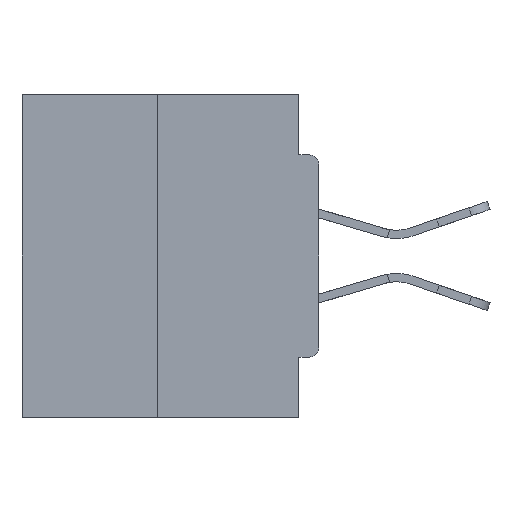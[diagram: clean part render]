
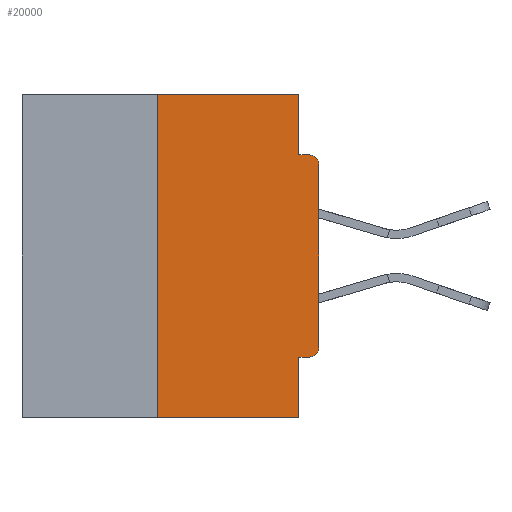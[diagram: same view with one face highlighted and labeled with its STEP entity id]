
A CAD part, left-side view. The second image highlights one B-rep face of the part: STEP entity #20000.
In plain terms, the highlighted planar face has unit normal (-1, 0, 0).
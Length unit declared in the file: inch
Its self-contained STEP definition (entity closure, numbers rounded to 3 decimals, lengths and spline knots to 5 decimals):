
#59 = DIRECTION ( 'NONE',  ( 0., 0., 1. ) ) ;
#1425 = VERTEX_POINT ( 'NONE', #32797 ) ;
#2034 = DIRECTION ( 'NONE',  ( 0., -1., 0. ) ) ;
#2106 = ORIENTED_EDGE ( 'NONE', *, *, #36228, .F. ) ;
#2875 = VECTOR ( 'NONE', #9010, 39.37008 ) ;
#3134 = DIRECTION ( 'NONE',  ( 0., 0., -1. ) ) ;
#3460 = VECTOR ( 'NONE', #59, 39.37008 ) ;
#3469 = EDGE_CURVE ( 'NONE', #21817, #31836, #18615, .T. ) ;
#4063 = CARTESIAN_POINT ( 'NONE',  ( 0., 0.25, -0.5 ) ) ;
#4413 = EDGE_CURVE ( 'NONE', #31836, #13114, #21707, .T. ) ;
#6212 = LINE ( 'NONE', #22505, #30817 ) ;
#6275 = EDGE_CURVE ( 'NONE', #23676, #8430, #10572, .T. ) ;
#6409 = CARTESIAN_POINT ( 'NONE',  ( 0., 0.031, 0. ) ) ;
#6540 = DIRECTION ( 'NONE',  ( -1., 0., 0. ) ) ;
#7031 = CARTESIAN_POINT ( 'NONE',  ( 0., 0.46, 0. ) ) ;
#7038 = DIRECTION ( 'NONE',  ( 0., 0., -1. ) ) ;
#7107 = ORIENTED_EDGE ( 'NONE', *, *, #3469, .F. ) ;
#7207 = CARTESIAN_POINT ( 'NONE',  ( 0., 0., -0.3915 ) ) ;
#8430 = VERTEX_POINT ( 'NONE', #20053 ) ;
#8773 = ORIENTED_EDGE ( 'NONE', *, *, #29819, .T. ) ;
#9010 = DIRECTION ( 'NONE',  ( 0., 0., -1. ) ) ;
#9365 = DIRECTION ( 'NONE',  ( 0., 0., -1. ) ) ;
#9433 = AXIS2_PLACEMENT_3D ( 'NONE', #29957, #6540, #9365 ) ;
#9590 = ORIENTED_EDGE ( 'NONE', *, *, #11597, .F. ) ;
#9687 = EDGE_CURVE ( 'NONE', #1425, #23676, #28152, .T. ) ;
#9873 = VECTOR ( 'NONE', #3134, 39.37008 ) ;
#9874 = EDGE_CURVE ( 'NONE', #1425, #29015, #23133, .T. ) ;
#10572 = LINE ( 'NONE', #11796, #2875 ) ;
#11354 = CARTESIAN_POINT ( 'NONE',  ( 0., 0., 0. ) ) ;
#11597 = EDGE_CURVE ( 'NONE', #22866, #21817, #6212, .T. ) ;
#11796 = CARTESIAN_POINT ( 'NONE',  ( 0., 0.031, -0.5 ) ) ;
#13114 = VERTEX_POINT ( 'NONE', #19167 ) ;
#13238 = CARTESIAN_POINT ( 'NONE',  ( 0., 0.031, -0.4065 ) ) ;
#13735 = DIRECTION ( 'NONE',  ( 0., -1., 0. ) ) ;
#14748 = CARTESIAN_POINT ( 'NONE',  ( 0., 0., -0.4065 ) ) ;
#15618 = DIRECTION ( 'NONE',  ( 1., 0., 0. ) ) ;
#15862 = DIRECTION ( 'NONE',  ( 0., 0., -1. ) ) ;
#15946 = DIRECTION ( 'NONE',  ( 0., -1., 0. ) ) ;
#16058 = VECTOR ( 'NONE', #15946, 39.37008 ) ;
#17193 = CARTESIAN_POINT ( 'NONE',  ( 0., 0.46, -0.5 ) ) ;
#17285 = VERTEX_POINT ( 'NONE', #30725 ) ;
#17289 = ORIENTED_EDGE ( 'NONE', *, *, #6275, .F. ) ;
#18047 = LINE ( 'NONE', #11354, #3460 ) ;
#18615 = LINE ( 'NONE', #18857, #20888 ) ;
#18857 = CARTESIAN_POINT ( 'NONE',  ( 0., 0.46, 0. ) ) ;
#18990 = ORIENTED_EDGE ( 'NONE', *, *, #27694, .T. ) ;
#19108 = ORIENTED_EDGE ( 'NONE', *, *, #4413, .F. ) ;
#19167 = CARTESIAN_POINT ( 'NONE',  ( 0., 0.031, -0.0935 ) ) ;
#20000 = ADVANCED_FACE ( 'NONE', ( #36616 ), #24073, .F. ) ;
#20053 = CARTESIAN_POINT ( 'NONE',  ( 0., 0.031, -0.5 ) ) ;
#20888 = VECTOR ( 'NONE', #2034, 39.37008 ) ;
#21130 = ORIENTED_EDGE ( 'NONE', *, *, #28886, .T. ) ;
#21433 = VECTOR ( 'NONE', #13735, 39.37008 ) ;
#21707 = LINE ( 'NONE', #6409, #9873 ) ;
#21817 = VERTEX_POINT ( 'NONE', #32088 ) ;
#22361 = DIRECTION ( 'NONE',  ( 0., 0., 1. ) ) ;
#22505 = CARTESIAN_POINT ( 'NONE',  ( 0., 0.25, 0. ) ) ;
#22832 = CARTESIAN_POINT ( 'NONE',  ( 0., 0., -0.1085 ) ) ;
#22866 = VERTEX_POINT ( 'NONE', #4063 ) ;
#23133 = CIRCLE ( 'NONE', #30347, 0.015 ) ;
#23594 = VECTOR ( 'NONE', #26531, 39.37008 ) ;
#23676 = VERTEX_POINT ( 'NONE', #13238 ) ;
#24073 = PLANE ( 'NONE',  #33627 ) ;
#24447 = DIRECTION ( 'NONE',  ( -1., 0., 0. ) ) ;
#26531 = DIRECTION ( 'NONE',  ( 0., 1., 0. ) ) ;
#27610 = CARTESIAN_POINT ( 'NONE',  ( 0., 0., -0.0935 ) ) ;
#27694 = EDGE_CURVE ( 'NONE', #28630, #17285, #32647, .T. ) ;
#27716 = ORIENTED_EDGE ( 'NONE', *, *, #9687, .F. ) ;
#28152 = LINE ( 'NONE', #14748, #23594 ) ;
#28220 = LINE ( 'NONE', #17193, #21433 ) ;
#28630 = VERTEX_POINT ( 'NONE', #22832 ) ;
#28886 = EDGE_CURVE ( 'NONE', #22866, #8430, #28220, .T. ) ;
#29015 = VERTEX_POINT ( 'NONE', #7207 ) ;
#29819 = EDGE_CURVE ( 'NONE', #29015, #28630, #18047, .T. ) ;
#29957 = CARTESIAN_POINT ( 'NONE',  ( 0., 0.015, -0.1085 ) ) ;
#30114 = LINE ( 'NONE', #27610, #16058 ) ;
#30347 = AXIS2_PLACEMENT_3D ( 'NONE', #36192, #24447, #7038 ) ;
#30725 = CARTESIAN_POINT ( 'NONE',  ( 0., 0.015, -0.0935 ) ) ;
#30817 = VECTOR ( 'NONE', #22361, 39.37008 ) ;
#31171 = CARTESIAN_POINT ( 'NONE',  ( 0., 0.031, 0. ) ) ;
#31836 = VERTEX_POINT ( 'NONE', #31171 ) ;
#32088 = CARTESIAN_POINT ( 'NONE',  ( 0., 0.25, 0. ) ) ;
#32647 = CIRCLE ( 'NONE', #9433, 0.015 ) ;
#32797 = CARTESIAN_POINT ( 'NONE',  ( 0., 0.015, -0.4065 ) ) ;
#33627 = AXIS2_PLACEMENT_3D ( 'NONE', #7031, #15618, #15862 ) ;
#35148 = EDGE_LOOP ( 'NONE', ( #7107, #9590, #21130, #17289, #27716, #35891, #8773, #18990, #2106, #19108 ) ) ;
#35891 = ORIENTED_EDGE ( 'NONE', *, *, #9874, .T. ) ;
#36192 = CARTESIAN_POINT ( 'NONE',  ( 0., 0.015, -0.3915 ) ) ;
#36228 = EDGE_CURVE ( 'NONE', #13114, #17285, #30114, .T. ) ;
#36616 = FACE_OUTER_BOUND ( 'NONE', #35148, .T. ) ;
